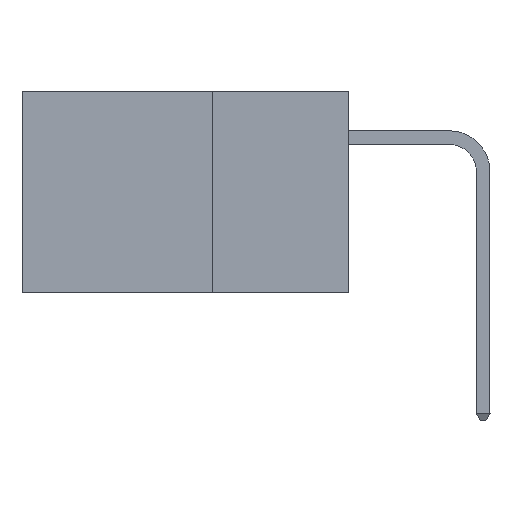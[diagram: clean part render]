
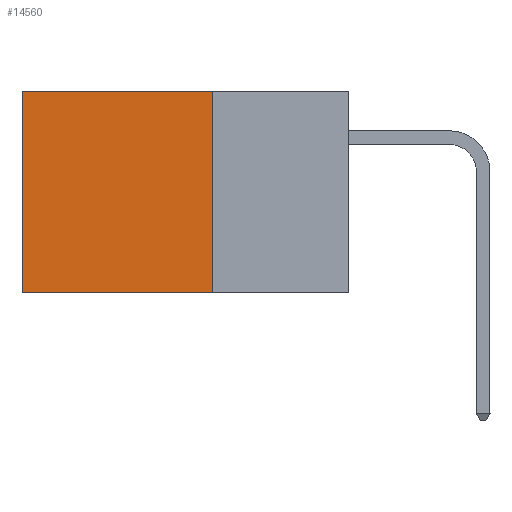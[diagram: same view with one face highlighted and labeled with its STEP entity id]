
A CAD part, left-side view. The second image highlights one B-rep face of the part: STEP entity #14560.
In plain terms, the highlighted planar face has unit normal (-1, 0, 0).
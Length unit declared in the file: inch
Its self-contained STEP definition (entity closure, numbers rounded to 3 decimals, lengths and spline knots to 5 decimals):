
#805 = CARTESIAN_POINT ( 'NONE',  ( 0.2875, 0.6, 0. ) ) ;
#1236 = VERTEX_POINT ( 'NONE', #33224 ) ;
#2070 = VECTOR ( 'NONE', #3903, 39.37008 ) ;
#2345 = VECTOR ( 'NONE', #16456, 39.37008 ) ;
#3591 = ORIENTED_EDGE ( 'NONE', *, *, #25513, .T. ) ;
#3903 = DIRECTION ( 'NONE',  ( 0., 1., 0. ) ) ;
#4105 = CARTESIAN_POINT ( 'NONE',  ( 0.2875, 0.25, 0. ) ) ;
#5597 = CARTESIAN_POINT ( 'NONE',  ( 0.2875, 0.25, -0.37 ) ) ;
#8309 = CARTESIAN_POINT ( 'NONE',  ( 0.2875, 0.6, -0.37 ) ) ;
#8650 = PLANE ( 'NONE',  #20299 ) ;
#11515 = CARTESIAN_POINT ( 'NONE',  ( 0.2875, 0.25, 0. ) ) ;
#12030 = CARTESIAN_POINT ( 'NONE',  ( 0.2875, 0.6, 0. ) ) ;
#12286 = LINE ( 'NONE', #24668, #35987 ) ;
#12736 = EDGE_LOOP ( 'NONE', ( #3591, #34780, #12763, #14305 ) ) ;
#12763 = ORIENTED_EDGE ( 'NONE', *, *, #39484, .F. ) ;
#14305 = ORIENTED_EDGE ( 'NONE', *, *, #36410, .T. ) ;
#14560 = ADVANCED_FACE ( 'NONE', ( #23506 ), #8650, .F. ) ;
#14961 = DIRECTION ( 'NONE',  ( 0., 0., -1. ) ) ;
#16456 = DIRECTION ( 'NONE',  ( 0., 0., -1. ) ) ;
#17419 = LINE ( 'NONE', #35691, #31444 ) ;
#17608 = DIRECTION ( 'NONE',  ( 0., 1., 0. ) ) ;
#17809 = DIRECTION ( 'NONE',  ( 1., 0., 0. ) ) ;
#18584 = DIRECTION ( 'NONE',  ( 0., 0., -1. ) ) ;
#20299 = AXIS2_PLACEMENT_3D ( 'NONE', #11515, #17809, #14961 ) ;
#22631 = EDGE_CURVE ( 'NONE', #28423, #30878, #17419, .T. ) ;
#23506 = FACE_OUTER_BOUND ( 'NONE', #12736, .T. ) ;
#24668 = CARTESIAN_POINT ( 'NONE',  ( 0.2875, 0.25, 0. ) ) ;
#25513 = EDGE_CURVE ( 'NONE', #39746, #30878, #28636, .T. ) ;
#28284 = LINE ( 'NONE', #4105, #2070 ) ;
#28423 = VERTEX_POINT ( 'NONE', #5597 ) ;
#28636 = LINE ( 'NONE', #805, #2345 ) ;
#30878 = VERTEX_POINT ( 'NONE', #8309 ) ;
#31444 = VECTOR ( 'NONE', #17608, 39.37008 ) ;
#33224 = CARTESIAN_POINT ( 'NONE',  ( 0.2875, 0.25, 0. ) ) ;
#34780 = ORIENTED_EDGE ( 'NONE', *, *, #22631, .F. ) ;
#35691 = CARTESIAN_POINT ( 'NONE',  ( 0.2875, 0.25, -0.37 ) ) ;
#35987 = VECTOR ( 'NONE', #18584, 39.37008 ) ;
#36410 = EDGE_CURVE ( 'NONE', #1236, #39746, #28284, .T. ) ;
#39484 = EDGE_CURVE ( 'NONE', #1236, #28423, #12286, .T. ) ;
#39746 = VERTEX_POINT ( 'NONE', #12030 ) ;
